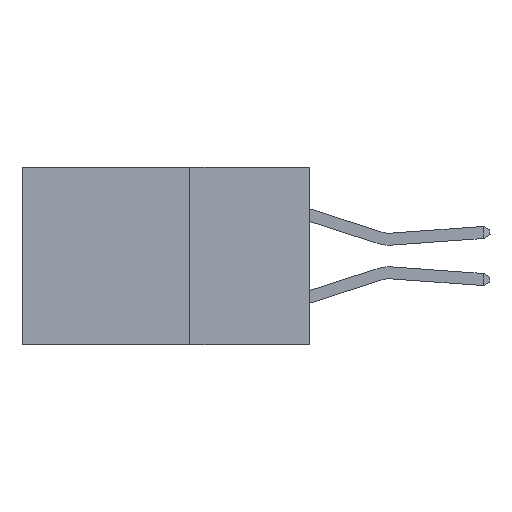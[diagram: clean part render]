
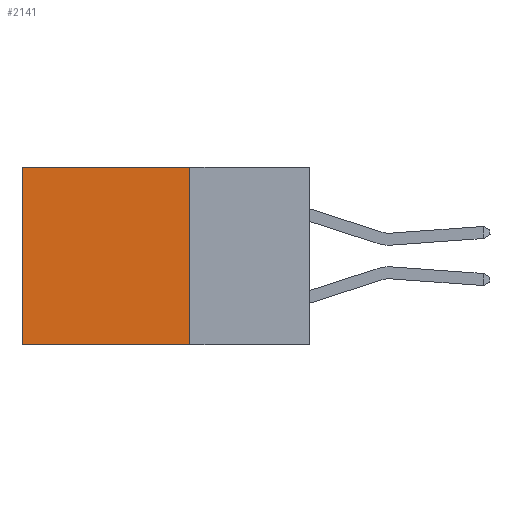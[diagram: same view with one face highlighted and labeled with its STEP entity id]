
A CAD part, left-side view. The second image highlights one B-rep face of the part: STEP entity #2141.
In plain terms, the highlighted planar face has unit normal (-1, 0, 0).
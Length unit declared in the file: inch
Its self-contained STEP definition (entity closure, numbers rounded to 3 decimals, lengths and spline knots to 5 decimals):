
#360 = CARTESIAN_POINT ( 'NONE',  ( 0.298, 0.6, -0.37 ) ) ;
#1264 = VERTEX_POINT ( 'NONE', #360 ) ;
#1948 = ORIENTED_EDGE ( 'NONE', *, *, #4349, .T. ) ;
#2141 = ADVANCED_FACE ( 'NONE', ( #19753 ), #9313, .F. ) ;
#2386 = VECTOR ( 'NONE', #11085, 39.37008 ) ;
#2455 = CARTESIAN_POINT ( 'NONE',  ( 0.298, 0.25, -0.37 ) ) ;
#3330 = CARTESIAN_POINT ( 'NONE',  ( 0.298, 0.25, 0. ) ) ;
#3494 = ORIENTED_EDGE ( 'NONE', *, *, #3689, .F. ) ;
#3689 = EDGE_CURVE ( 'NONE', #15248, #1264, #16012, .T. ) ;
#4349 = EDGE_CURVE ( 'NONE', #10522, #5243, #7864, .T. ) ;
#4371 = EDGE_LOOP ( 'NONE', ( #12682, #3494, #15258, #1948 ) ) ;
#5243 = VERTEX_POINT ( 'NONE', #13824 ) ;
#6285 = LINE ( 'NONE', #18042, #9482 ) ;
#6301 = DIRECTION ( 'NONE',  ( 0., 0., -1. ) ) ;
#6407 = DIRECTION ( 'NONE',  ( 0., 1., 0. ) ) ;
#6865 = LINE ( 'NONE', #16008, #2386 ) ;
#7630 = VECTOR ( 'NONE', #6407, 39.37008 ) ;
#7864 = LINE ( 'NONE', #3330, #16243 ) ;
#9313 = PLANE ( 'NONE',  #12835 ) ;
#9456 = CARTESIAN_POINT ( 'NONE',  ( 0.298, 0.25, 0. ) ) ;
#9482 = VECTOR ( 'NONE', #6301, 39.37008 ) ;
#10522 = VERTEX_POINT ( 'NONE', #17707 ) ;
#10527 = EDGE_CURVE ( 'NONE', #5243, #1264, #6865, .T. ) ;
#11085 = DIRECTION ( 'NONE',  ( 0., 0., -1. ) ) ;
#11328 = EDGE_CURVE ( 'NONE', #10522, #15248, #6285, .T. ) ;
#11866 = DIRECTION ( 'NONE',  ( 1., 0., 0. ) ) ;
#11869 = DIRECTION ( 'NONE',  ( 0., 0., -1. ) ) ;
#12682 = ORIENTED_EDGE ( 'NONE', *, *, #10527, .T. ) ;
#12835 = AXIS2_PLACEMENT_3D ( 'NONE', #9456, #11866, #11869 ) ;
#13824 = CARTESIAN_POINT ( 'NONE',  ( 0.298, 0.6, 0. ) ) ;
#14745 = CARTESIAN_POINT ( 'NONE',  ( 0.298, 0.25, -0.37 ) ) ;
#15248 = VERTEX_POINT ( 'NONE', #2455 ) ;
#15258 = ORIENTED_EDGE ( 'NONE', *, *, #11328, .F. ) ;
#16008 = CARTESIAN_POINT ( 'NONE',  ( 0.298, 0.6, 0. ) ) ;
#16012 = LINE ( 'NONE', #14745, #7630 ) ;
#16243 = VECTOR ( 'NONE', #18438, 39.37008 ) ;
#17707 = CARTESIAN_POINT ( 'NONE',  ( 0.298, 0.25, 0. ) ) ;
#18042 = CARTESIAN_POINT ( 'NONE',  ( 0.298, 0.25, 0. ) ) ;
#18438 = DIRECTION ( 'NONE',  ( 0., 1., 0. ) ) ;
#19753 = FACE_OUTER_BOUND ( 'NONE', #4371, .T. ) ;
